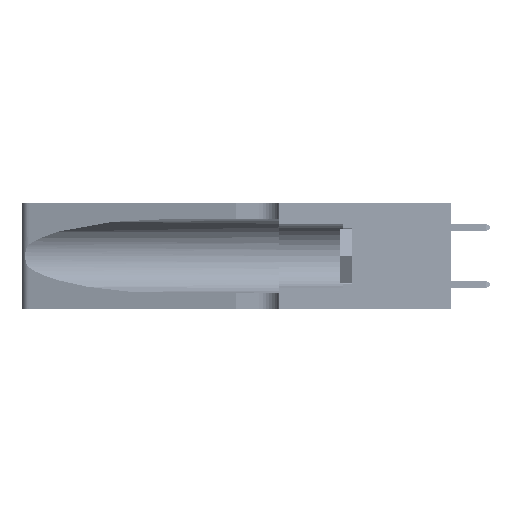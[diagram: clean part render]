
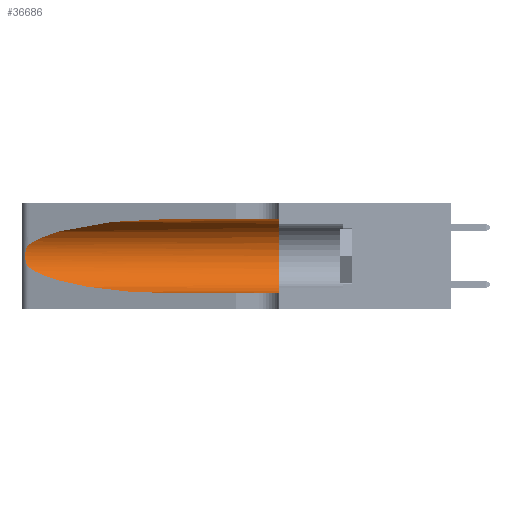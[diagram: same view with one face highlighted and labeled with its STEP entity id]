
A CAD part, left-side view. The second image highlights one B-rep face of the part: STEP entity #36686.
In plain terms, the highlighted cylindrical face has radius 3.308 mm (diameter 6.617 mm), a partial arc.
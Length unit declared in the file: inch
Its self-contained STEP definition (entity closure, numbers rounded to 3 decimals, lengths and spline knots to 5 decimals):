
#786 = CARTESIAN_POINT ( 'NONE',  ( 0.26075, 1.23896, 0.178 ) ) ;
#1030 = CYLINDRICAL_SURFACE ( 'NONE', #36693, 0.13025 ) ;
#1349 = VERTEX_POINT ( 'NONE', #18202 ) ;
#4192 = CIRCLE ( 'NONE', #12315, 0.13025 ) ;
#8208 = CARTESIAN_POINT ( 'NONE',  ( 0.25487, 1.22718, 0.14631 ) ) ;
#8537 = EDGE_CURVE ( 'NONE', #39492, #22519, #25637, .T. ) ;
#8538 = CARTESIAN_POINT ( 'NONE',  ( 0.25487, 1.22718, 0.22369 ) ) ;
#8701 = CARTESIAN_POINT ( 'NONE',  ( 0.26018, 1.23835, 0.19895 ) ) ;
#8863 = CARTESIAN_POINT ( 'NONE',  ( 0.26075, 1.23896, 0.19203 ) ) ;
#10214 = CARTESIAN_POINT ( 'NONE',  ( 0.1305, 0.72297, 0.31525 ) ) ;
#10570 = DIRECTION ( 'NONE',  ( 0., -1., 0. ) ) ;
#11695 = LINE ( 'NONE', #29025, #24112 ) ;
#12315 = AXIS2_PLACEMENT_3D ( 'NONE', #42300, #16090, #19555 ) ;
#12605 = ORIENTED_EDGE ( 'NONE', *, *, #8537, .T. ) ;
#13146 = ORIENTED_EDGE ( 'NONE', *, *, #23236, .F. ) ;
#13863 = DIRECTION ( 'NONE',  ( 0., -1., 0. ) ) ;
#15109 = VERTEX_POINT ( 'NONE', #15922 ) ;
#15922 = CARTESIAN_POINT ( 'NONE',  ( 0.25487, 1.22718, 0.22369 ) ) ;
#16090 = DIRECTION ( 'NONE',  ( 0., 1., 0. ) ) ;
#16239 = CARTESIAN_POINT ( 'NONE',  ( 0.25639, 1.23186, 0.15144 ) ) ;
#16845 = B_SPLINE_CURVE_WITH_KNOTS ( 'NONE', 3,
 ( #8538, #31260, #19546, #23358, #30758, #8701, #8863, #786, #35203, #23850, #46596, #16239, #42791, #8208 ),
 .UNSPECIFIED., .F., .F.,
 ( 4, 2, 2, 2, 2, 2, 4 ),
 ( 0., 0.00027, 0.00053, 0.00107, 0.0016, 0.00187, 0.00214 ),
 .UNSPECIFIED. ) ;
#17404 = CARTESIAN_POINT ( 'NONE',  ( 0.25487, 1.22718, 0.14631 ) ) ;
#17654 = CARTESIAN_POINT ( 'NONE',  ( 0.1305, 1.61858, 0.185 ) ) ;
#18202 = CARTESIAN_POINT ( 'NONE',  ( 0.1305, 0.35, 0.05475 ) ) ;
#19546 = CARTESIAN_POINT ( 'NONE',  ( 0.25639, 1.23184, 0.21858 ) ) ;
#19555 = DIRECTION ( 'NONE',  ( 0., 0., 1. ) ) ;
#20287 = CARTESIAN_POINT ( 'NONE',  ( 0.1305, 1.61858, 0.05475 ) ) ;
#20451 = DIRECTION ( 'NONE',  ( 0., -1., 0. ) ) ;
#21216 = CARTESIAN_POINT ( 'NONE',  ( 0.2373, 1.15595, 0.08982 ) ) ;
#21314 = DIRECTION ( 'NONE',  ( 0., 0., -1. ) ) ;
#21373 = EDGE_CURVE ( 'NONE', #15109, #39492, #16845, .T. ) ;
#22519 = VERTEX_POINT ( 'NONE', #22587 ) ;
#22526 = ORIENTED_EDGE ( 'NONE', *, *, #23594, .T. ) ;
#22587 = CARTESIAN_POINT ( 'NONE',  ( 0.1305, 0.72297, 0.05475 ) ) ;
#23236 = EDGE_CURVE ( 'NONE', #31064, #1349, #4192, .T. ) ;
#23358 = CARTESIAN_POINT ( 'NONE',  ( 0.25787, 1.23484, 0.2124 ) ) ;
#23594 = EDGE_CURVE ( 'NONE', #22519, #1349, #46626, .T. ) ;
#23850 = CARTESIAN_POINT ( 'NONE',  ( 0.25856, 1.23593, 0.16098 ) ) ;
#24112 = VECTOR ( 'NONE', #13863, 39.37008 ) ;
#24193 = VERTEX_POINT ( 'NONE', #42314 ) ;
#24718 = ORIENTED_EDGE ( 'NONE', *, *, #21373, .T. ) ;
#25637 =( BOUNDED_CURVE ( )  B_SPLINE_CURVE ( 3, ( #17404, #21216, #47604, #36517 ),
 .UNSPECIFIED., .F., .F. ) 
 B_SPLINE_CURVE_WITH_KNOTS ( ( 4, 4 ),
 ( 3.44316, 4.71239 ),
 .UNSPECIFIED. ) 
 CURVE ( )  GEOMETRIC_REPRESENTATION_ITEM ( )  RATIONAL_B_SPLINE_CURVE ( ( 1., 0.87, 0.87, 1. ) ) 
 REPRESENTATION_ITEM ( '' )  );
#26497 = ORIENTED_EDGE ( 'NONE', *, *, #30227, .T. ) ;
#29025 = CARTESIAN_POINT ( 'NONE',  ( 0.1305, 1.61858, 0.31525 ) ) ;
#29388 = CARTESIAN_POINT ( 'NONE',  ( 0.1305, 0.35, 0.31525 ) ) ;
#30227 = EDGE_CURVE ( 'NONE', #24193, #15109, #47705, .T. ) ;
#30758 = CARTESIAN_POINT ( 'NONE',  ( 0.25854, 1.2359, 0.20912 ) ) ;
#31064 = VERTEX_POINT ( 'NONE', #29388 ) ;
#31260 = CARTESIAN_POINT ( 'NONE',  ( 0.25555, 1.22994, 0.2215 ) ) ;
#31715 = FACE_OUTER_BOUND ( 'NONE', #33809, .T. ) ;
#32618 = CARTESIAN_POINT ( 'NONE',  ( 0.2373, 1.15595, 0.28018 ) ) ;
#32941 = CARTESIAN_POINT ( 'NONE',  ( 0.18966, 0.96281, 0.31525 ) ) ;
#33809 = EDGE_LOOP ( 'NONE', ( #26497, #24718, #12605, #22526, #13146, #38976 ) ) ;
#34997 = CARTESIAN_POINT ( 'NONE',  ( 0.25487, 1.22718, 0.14631 ) ) ;
#35203 = CARTESIAN_POINT ( 'NONE',  ( 0.26017, 1.23833, 0.17102 ) ) ;
#36089 = EDGE_CURVE ( 'NONE', #24193, #31064, #11695, .T. ) ;
#36517 = CARTESIAN_POINT ( 'NONE',  ( 0.1305, 0.72297, 0.05475 ) ) ;
#36686 = ADVANCED_FACE ( 'NONE', ( #31715 ), #1030, .F. ) ;
#36693 = AXIS2_PLACEMENT_3D ( 'NONE', #17654, #10570, #21314 ) ;
#38976 = ORIENTED_EDGE ( 'NONE', *, *, #36089, .F. ) ;
#39492 = VERTEX_POINT ( 'NONE', #34997 ) ;
#40513 = CARTESIAN_POINT ( 'NONE',  ( 0.25487, 1.22718, 0.22369 ) ) ;
#42300 = CARTESIAN_POINT ( 'NONE',  ( 0.1305, 0.35, 0.185 ) ) ;
#42314 = CARTESIAN_POINT ( 'NONE',  ( 0.1305, 0.72297, 0.31525 ) ) ;
#42791 = CARTESIAN_POINT ( 'NONE',  ( 0.25555, 1.22993, 0.14849 ) ) ;
#45420 = VECTOR ( 'NONE', #20451, 39.37008 ) ;
#46596 = CARTESIAN_POINT ( 'NONE',  ( 0.25789, 1.23486, 0.15765 ) ) ;
#46626 = LINE ( 'NONE', #20287, #45420 ) ;
#47604 = CARTESIAN_POINT ( 'NONE',  ( 0.18966, 0.96281, 0.05475 ) ) ;
#47705 =( BOUNDED_CURVE ( )  B_SPLINE_CURVE ( 3, ( #10214, #32941, #32618, #40513 ),
 .UNSPECIFIED., .F., .T. ) 
 B_SPLINE_CURVE_WITH_KNOTS ( ( 4, 4 ),
 ( 1.5708, 2.84003 ),
 .UNSPECIFIED. ) 
 CURVE ( )  GEOMETRIC_REPRESENTATION_ITEM ( )  RATIONAL_B_SPLINE_CURVE ( ( 1., 0.87, 0.87, 1. ) ) 
 REPRESENTATION_ITEM ( '' )  );
